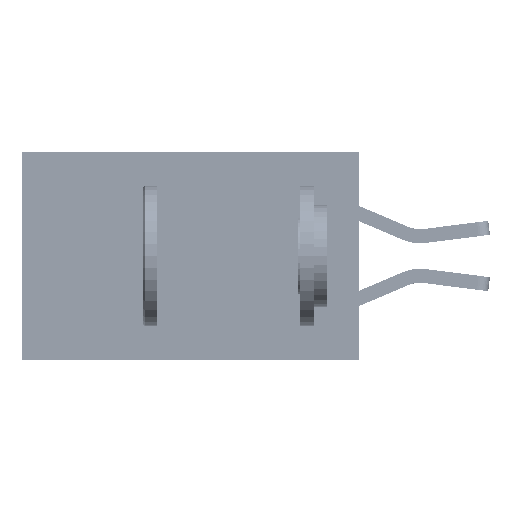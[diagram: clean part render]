
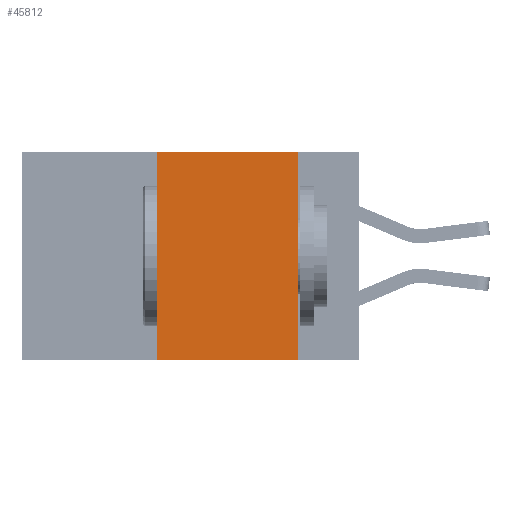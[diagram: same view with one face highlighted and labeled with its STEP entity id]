
A CAD part, left-side view. The second image highlights one B-rep face of the part: STEP entity #45812.
In plain terms, the highlighted planar face has unit normal (-1, 0, 0).
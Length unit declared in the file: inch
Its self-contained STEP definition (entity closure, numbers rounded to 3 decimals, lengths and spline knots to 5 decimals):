
#361 = CARTESIAN_POINT ( 'NONE',  ( 0., 0.36, -0.37 ) ) ;
#416 = EDGE_CURVE ( 'NONE', #12625, #15549, #23494, .T. ) ;
#943 = CARTESIAN_POINT ( 'NONE',  ( 0., 0.36, 0. ) ) ;
#2006 = DIRECTION ( 'NONE',  ( 0., 0., 1. ) ) ;
#3206 = VERTEX_POINT ( 'NONE', #943 ) ;
#5932 = ORIENTED_EDGE ( 'NONE', *, *, #20301, .F. ) ;
#5952 = CARTESIAN_POINT ( 'NONE',  ( 0., 0.11, 0. ) ) ;
#6847 = AXIS2_PLACEMENT_3D ( 'NONE', #34568, #22405, #9895 ) ;
#7738 = DIRECTION ( 'NONE',  ( 0., -1., 0. ) ) ;
#8217 = DIRECTION ( 'NONE',  ( 0., -1., 0. ) ) ;
#8709 = ORIENTED_EDGE ( 'NONE', *, *, #30629, .F. ) ;
#9895 = DIRECTION ( 'NONE',  ( 0., 0., -1. ) ) ;
#10190 = EDGE_LOOP ( 'NONE', ( #5932, #8709, #35269, #29858 ) ) ;
#11084 = LINE ( 'NONE', #53490, #30573 ) ;
#12625 = VERTEX_POINT ( 'NONE', #361 ) ;
#14101 = DIRECTION ( 'NONE',  ( 0., 0., -1. ) ) ;
#15549 = VERTEX_POINT ( 'NONE', #26120 ) ;
#20301 = EDGE_CURVE ( 'NONE', #33036, #15549, #34728, .T. ) ;
#20610 = CARTESIAN_POINT ( 'NONE',  ( 0., 0.6, -0.37 ) ) ;
#22405 = DIRECTION ( 'NONE',  ( 1., 0., 0. ) ) ;
#23494 = LINE ( 'NONE', #20610, #46207 ) ;
#23808 = FACE_OUTER_BOUND ( 'NONE', #10190, .T. ) ;
#26120 = CARTESIAN_POINT ( 'NONE',  ( 0., 0.11, -0.37 ) ) ;
#29858 = ORIENTED_EDGE ( 'NONE', *, *, #416, .T. ) ;
#30510 = LINE ( 'NONE', #38919, #38234 ) ;
#30573 = VECTOR ( 'NONE', #8217, 39.37008 ) ;
#30629 = EDGE_CURVE ( 'NONE', #3206, #33036, #11084, .T. ) ;
#33036 = VERTEX_POINT ( 'NONE', #34710 ) ;
#34568 = CARTESIAN_POINT ( 'NONE',  ( 0., 0.6, 0. ) ) ;
#34710 = CARTESIAN_POINT ( 'NONE',  ( 0., 0.11, 0. ) ) ;
#34728 = LINE ( 'NONE', #5952, #52821 ) ;
#34928 = PLANE ( 'NONE',  #6847 ) ;
#35269 = ORIENTED_EDGE ( 'NONE', *, *, #50398, .F. ) ;
#38234 = VECTOR ( 'NONE', #2006, 39.37008 ) ;
#38919 = CARTESIAN_POINT ( 'NONE',  ( 0., 0.36, 0. ) ) ;
#45812 = ADVANCED_FACE ( 'NONE', ( #23808 ), #34928, .F. ) ;
#46207 = VECTOR ( 'NONE', #7738, 39.37008 ) ;
#50398 = EDGE_CURVE ( 'NONE', #12625, #3206, #30510, .T. ) ;
#52821 = VECTOR ( 'NONE', #14101, 39.37008 ) ;
#53490 = CARTESIAN_POINT ( 'NONE',  ( 0., 0.6, 0. ) ) ;
